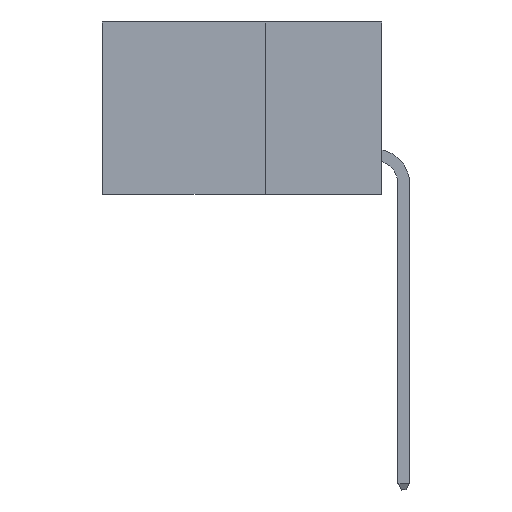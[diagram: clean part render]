
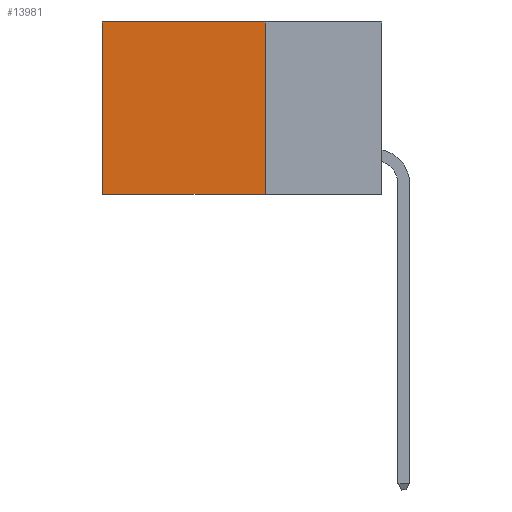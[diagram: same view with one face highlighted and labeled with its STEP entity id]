
A CAD part, left-side view. The second image highlights one B-rep face of the part: STEP entity #13981.
In plain terms, the highlighted planar face has unit normal (-1, 0, 0).
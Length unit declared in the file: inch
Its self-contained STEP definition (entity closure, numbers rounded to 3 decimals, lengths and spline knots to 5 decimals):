
#85 = FACE_OUTER_BOUND ( 'NONE', #19949, .T. ) ;
#826 = CARTESIAN_POINT ( 'NONE',  ( 0.2875, 0.6, 0. ) ) ;
#1673 = DIRECTION ( 'NONE',  ( 1., 0., 0. ) ) ;
#2194 = CARTESIAN_POINT ( 'NONE',  ( 0.2875, 0.25, -0.37 ) ) ;
#2262 = CARTESIAN_POINT ( 'NONE',  ( 0.2875, 0.25, -0.37 ) ) ;
#2546 = AXIS2_PLACEMENT_3D ( 'NONE', #14017, #1673, #21280 ) ;
#2773 = LINE ( 'NONE', #2194, #15196 ) ;
#3088 = VERTEX_POINT ( 'NONE', #15656 ) ;
#3474 = DIRECTION ( 'NONE',  ( 0., 1., 0. ) ) ;
#5807 = ORIENTED_EDGE ( 'NONE', *, *, #13890, .F. ) ;
#6479 = LINE ( 'NONE', #15514, #12558 ) ;
#8030 = VERTEX_POINT ( 'NONE', #22204 ) ;
#10043 = ORIENTED_EDGE ( 'NONE', *, *, #10955, .T. ) ;
#10140 = DIRECTION ( 'NONE',  ( 0., 0., -1. ) ) ;
#10937 = VECTOR ( 'NONE', #3474, 39.37008 ) ;
#10955 = EDGE_CURVE ( 'NONE', #11572, #8030, #22912, .T. ) ;
#11572 = VERTEX_POINT ( 'NONE', #15748 ) ;
#12558 = VECTOR ( 'NONE', #10140, 39.37008 ) ;
#13099 = VECTOR ( 'NONE', #13174, 39.37008 ) ;
#13174 = DIRECTION ( 'NONE',  ( 0., 0., -1. ) ) ;
#13739 = EDGE_CURVE ( 'NONE', #8030, #3088, #19793, .T. ) ;
#13890 = EDGE_CURVE ( 'NONE', #11572, #15450, #6479, .T. ) ;
#13981 = ADVANCED_FACE ( 'NONE', ( #85 ), #20961, .F. ) ;
#14017 = CARTESIAN_POINT ( 'NONE',  ( 0.2875, 0.25, 0. ) ) ;
#15196 = VECTOR ( 'NONE', #16273, 39.37008 ) ;
#15450 = VERTEX_POINT ( 'NONE', #2262 ) ;
#15514 = CARTESIAN_POINT ( 'NONE',  ( 0.2875, 0.25, 0. ) ) ;
#15656 = CARTESIAN_POINT ( 'NONE',  ( 0.2875, 0.6, -0.37 ) ) ;
#15748 = CARTESIAN_POINT ( 'NONE',  ( 0.2875, 0.25, 0. ) ) ;
#16273 = DIRECTION ( 'NONE',  ( 0., 1., 0. ) ) ;
#17216 = EDGE_CURVE ( 'NONE', #15450, #3088, #2773, .T. ) ;
#18431 = ORIENTED_EDGE ( 'NONE', *, *, #13739, .T. ) ;
#18735 = CARTESIAN_POINT ( 'NONE',  ( 0.2875, 0.25, 0. ) ) ;
#19793 = LINE ( 'NONE', #826, #13099 ) ;
#19949 = EDGE_LOOP ( 'NONE', ( #18431, #20952, #5807, #10043 ) ) ;
#20952 = ORIENTED_EDGE ( 'NONE', *, *, #17216, .F. ) ;
#20961 = PLANE ( 'NONE',  #2546 ) ;
#21280 = DIRECTION ( 'NONE',  ( 0., 0., -1. ) ) ;
#22204 = CARTESIAN_POINT ( 'NONE',  ( 0.2875, 0.6, 0. ) ) ;
#22912 = LINE ( 'NONE', #18735, #10937 ) ;
